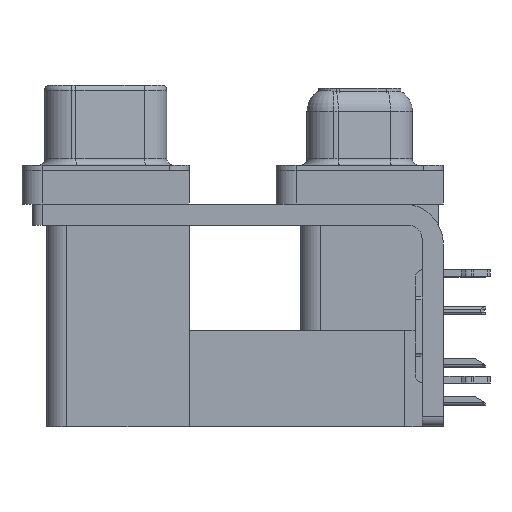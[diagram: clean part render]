
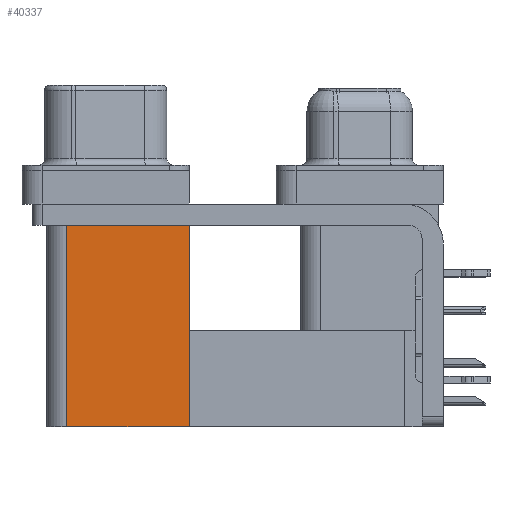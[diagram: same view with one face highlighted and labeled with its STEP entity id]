
A CAD part, left-side view. The second image highlights one B-rep face of the part: STEP entity #40337.
In plain terms, the highlighted planar face has unit normal (-1, 0, 0).
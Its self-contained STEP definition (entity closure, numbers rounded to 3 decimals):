
#751 = CARTESIAN_POINT ( 'NONE',  ( 3.765, 12.775, -2.5 ) ) ;
#962 = ORIENTED_EDGE ( 'NONE', *, *, #21987, .T. ) ;
#1339 = ORIENTED_EDGE ( 'NONE', *, *, #45356, .T. ) ;
#6619 = CARTESIAN_POINT ( 'NONE',  ( 3.765, 12.775, -19.2 ) ) ;
#10363 = ORIENTED_EDGE ( 'NONE', *, *, #41806, .F. ) ;
#13353 = DIRECTION ( 'NONE',  ( 0., 0., 1. ) ) ;
#13437 = EDGE_LOOP ( 'NONE', ( #962, #10363, #17495, #1339 ) ) ;
#14944 = VERTEX_POINT ( 'NONE', #37184 ) ;
#15807 = VERTEX_POINT ( 'NONE', #751 ) ;
#16590 = DIRECTION ( 'NONE',  ( 0., 1., 0. ) ) ;
#16876 = CARTESIAN_POINT ( 'NONE',  ( 3.765, 21.975, -19.2 ) ) ;
#17495 = ORIENTED_EDGE ( 'NONE', *, *, #39852, .F. ) ;
#18877 = CARTESIAN_POINT ( 'NONE',  ( 3.765, 12.775, -19.2 ) ) ;
#20936 = PLANE ( 'NONE',  #34580 ) ;
#20991 = DIRECTION ( 'NONE',  ( 0., 1., 0. ) ) ;
#21858 = FACE_OUTER_BOUND ( 'NONE', #13437, .T. ) ;
#21987 = EDGE_CURVE ( 'NONE', #15807, #23560, #45606, .T. ) ;
#23560 = VERTEX_POINT ( 'NONE', #41057 ) ;
#24185 = LINE ( 'NONE', #16876, #30839 ) ;
#25955 = VERTEX_POINT ( 'NONE', #27342 ) ;
#27342 = CARTESIAN_POINT ( 'NONE',  ( 3.765, 12.775, -19.2 ) ) ;
#28465 = CARTESIAN_POINT ( 'NONE',  ( 3.765, 12.775, -19.2 ) ) ;
#29954 = LINE ( 'NONE', #18877, #37116 ) ;
#30839 = VECTOR ( 'NONE', #13353, 1000. ) ;
#32253 = DIRECTION ( 'NONE',  ( 1., 0., 0. ) ) ;
#34580 = AXIS2_PLACEMENT_3D ( 'NONE', #28465, #32253, #42868 ) ;
#36086 = VECTOR ( 'NONE', #20991, 1000. ) ;
#36818 = DIRECTION ( 'NONE',  ( 0., 0., 1. ) ) ;
#37116 = VECTOR ( 'NONE', #36818, 1000. ) ;
#37184 = CARTESIAN_POINT ( 'NONE',  ( 3.765, 21.975, -19.2 ) ) ;
#37838 = CARTESIAN_POINT ( 'NONE',  ( 3.765, 12.775, -2.5 ) ) ;
#39852 = EDGE_CURVE ( 'NONE', #25955, #14944, #42457, .T. ) ;
#40337 = ADVANCED_FACE ( 'NONE', ( #21858 ), #20936, .F. ) ;
#41057 = CARTESIAN_POINT ( 'NONE',  ( 3.765, 21.975, -2.5 ) ) ;
#41806 = EDGE_CURVE ( 'NONE', #14944, #23560, #24185, .T. ) ;
#42457 = LINE ( 'NONE', #6619, #36086 ) ;
#42868 = DIRECTION ( 'NONE',  ( 0., 0., -1. ) ) ;
#45356 = EDGE_CURVE ( 'NONE', #25955, #15807, #29954, .T. ) ;
#45606 = LINE ( 'NONE', #37838, #46457 ) ;
#46457 = VECTOR ( 'NONE', #16590, 1000. ) ;
